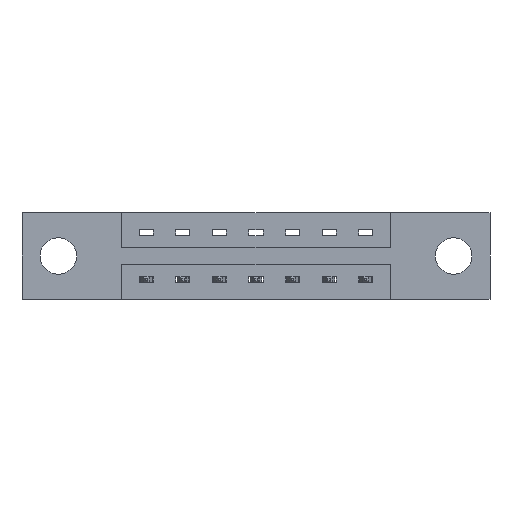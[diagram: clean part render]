
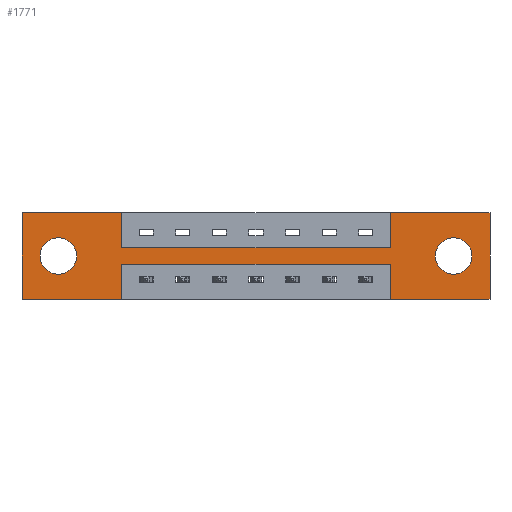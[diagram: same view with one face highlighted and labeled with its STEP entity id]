
A CAD part, front view. The second image highlights one B-rep face of the part: STEP entity #1771.
In plain terms, the highlighted planar face has unit normal (0, -1, 0).
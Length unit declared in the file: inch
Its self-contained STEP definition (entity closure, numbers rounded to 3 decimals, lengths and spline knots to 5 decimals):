
#3 = VERTEX_POINT ( 'NONE', #6277 ) ;
#59 = ORIENTED_EDGE ( 'NONE', *, *, #99, .F. ) ;
#99 = EDGE_CURVE ( 'NONE', #6538, #8846, #1955, .T. ) ;
#178 = AXIS2_PLACEMENT_3D ( 'NONE', #4753, #2896, #6939 ) ;
#201 = EDGE_CURVE ( 'NONE', #2395, #3969, #7067, .T. ) ;
#270 = ORIENTED_EDGE ( 'NONE', *, *, #6756, .T. ) ;
#272 = VECTOR ( 'NONE', #6194, 39.37008 ) ;
#516 = DIRECTION ( 'NONE',  ( 1., 0., 0. ) ) ;
#814 = EDGE_CURVE ( 'NONE', #7481, #3927, #6396, .T. ) ;
#838 = FACE_BOUND ( 'NONE', #1174, .T. ) ;
#1009 = CARTESIAN_POINT ( 'NONE',  ( 0.425, 0., 0. ) ) ;
#1174 = EDGE_LOOP ( 'NONE', ( #270, #1227 ) ) ;
#1227 = ORIENTED_EDGE ( 'NONE', *, *, #9350, .T. ) ;
#1290 = DIRECTION ( 'NONE',  ( 0., 0., -1. ) ) ;
#1318 = CARTESIAN_POINT ( 'NONE',  ( 0., 0., 0. ) ) ;
#1406 = VERTEX_POINT ( 'NONE', #3930 ) ;
#1412 = EDGE_CURVE ( 'NONE', #8813, #9386, #3619, .T. ) ;
#1627 = LINE ( 'NONE', #5317, #9279 ) ;
#1650 = CIRCLE ( 'NONE', #178, 0.078 ) ;
#1763 = CARTESIAN_POINT ( 'NONE',  ( 1.843, 0., -0.107 ) ) ;
#1771 = ADVANCED_FACE ( 'NONE', ( #838, #4845, #8669 ), #6172, .T. ) ;
#1793 = LINE ( 'NONE', #5709, #2046 ) ;
#1825 = CARTESIAN_POINT ( 'NONE',  ( 1.573, 0., -0.22 ) ) ;
#1839 = VERTEX_POINT ( 'NONE', #8819 ) ;
#1882 = VERTEX_POINT ( 'NONE', #7602 ) ;
#1948 = AXIS2_PLACEMENT_3D ( 'NONE', #8360, #5948, #5846 ) ;
#1955 = LINE ( 'NONE', #7317, #9540 ) ;
#1995 = VERTEX_POINT ( 'NONE', #5194 ) ;
#2046 = VECTOR ( 'NONE', #4275, 39.37008 ) ;
#2153 = VECTOR ( 'NONE', #2282, 39.37008 ) ;
#2155 = EDGE_CURVE ( 'NONE', #1882, #9260, #1650, .T. ) ;
#2158 = CARTESIAN_POINT ( 'NONE',  ( 0., 0., -0.37 ) ) ;
#2205 = ORIENTED_EDGE ( 'NONE', *, *, #6472, .F. ) ;
#2218 = CARTESIAN_POINT ( 'NONE',  ( 0., 0., 0. ) ) ;
#2282 = DIRECTION ( 'NONE',  ( -1., 0., 0. ) ) ;
#2288 = CARTESIAN_POINT ( 'NONE',  ( 0.155, 0., -0.185 ) ) ;
#2307 = CARTESIAN_POINT ( 'NONE',  ( 1.573, 0., -0.37 ) ) ;
#2395 = VERTEX_POINT ( 'NONE', #6501 ) ;
#2566 = ORIENTED_EDGE ( 'NONE', *, *, #2155, .T. ) ;
#2567 = DIRECTION ( 'NONE',  ( 0., 1., 0. ) ) ;
#2609 = CARTESIAN_POINT ( 'NONE',  ( 0.425, 0., -0.15 ) ) ;
#2838 = CIRCLE ( 'NONE', #5647, 0.078 ) ;
#2896 = DIRECTION ( 'NONE',  ( 0., 1., 0. ) ) ;
#2919 = EDGE_CURVE ( 'NONE', #1995, #6242, #9632, .T. ) ;
#3055 = DIRECTION ( 'NONE',  ( 0., 0., 1. ) ) ;
#3143 = VECTOR ( 'NONE', #8199, 39.37008 ) ;
#3165 = ORIENTED_EDGE ( 'NONE', *, *, #3813, .F. ) ;
#3193 = DIRECTION ( 'NONE',  ( 1., 0., 0. ) ) ;
#3371 = VECTOR ( 'NONE', #9126, 39.37008 ) ;
#3372 = EDGE_CURVE ( 'NONE', #8846, #1839, #9209, .T. ) ;
#3468 = CARTESIAN_POINT ( 'NONE',  ( 0.425, 0., -0.22 ) ) ;
#3476 = ORIENTED_EDGE ( 'NONE', *, *, #1412, .F. ) ;
#3619 = LINE ( 'NONE', #3981, #9204 ) ;
#3813 = EDGE_CURVE ( 'NONE', #1406, #2395, #1793, .T. ) ;
#3874 = VECTOR ( 'NONE', #7718, 39.37008 ) ;
#3924 = CIRCLE ( 'NONE', #1948, 0.078 ) ;
#3927 = VERTEX_POINT ( 'NONE', #9641 ) ;
#3930 = CARTESIAN_POINT ( 'NONE',  ( 1.573, 0., -0.15 ) ) ;
#3969 = VERTEX_POINT ( 'NONE', #8452 ) ;
#3981 = CARTESIAN_POINT ( 'NONE',  ( 0.425, 0., 0. ) ) ;
#4002 = CARTESIAN_POINT ( 'NONE',  ( 0.155, 0., -0.263 ) ) ;
#4010 = EDGE_LOOP ( 'NONE', ( #2566, #9467 ) ) ;
#4027 = CARTESIAN_POINT ( 'NONE',  ( 0., 0., 0. ) ) ;
#4216 = LINE ( 'NONE', #2158, #2153 ) ;
#4275 = DIRECTION ( 'NONE',  ( 0., 0., 1. ) ) ;
#4365 = EDGE_CURVE ( 'NONE', #1839, #7481, #4216, .T. ) ;
#4553 = LINE ( 'NONE', #2307, #272 ) ;
#4746 = CIRCLE ( 'NONE', #5968, 0.078 ) ;
#4753 = CARTESIAN_POINT ( 'NONE',  ( 0.155, 0., -0.185 ) ) ;
#4845 = FACE_BOUND ( 'NONE', #4010, .T. ) ;
#4879 = VECTOR ( 'NONE', #3193, 39.37008 ) ;
#5011 = LINE ( 'NONE', #2218, #3143 ) ;
#5044 = DIRECTION ( 'NONE',  ( 0., -1., 0. ) ) ;
#5111 = ORIENTED_EDGE ( 'NONE', *, *, #814, .F. ) ;
#5194 = CARTESIAN_POINT ( 'NONE',  ( 1.998, 0., -0.37 ) ) ;
#5252 = ORIENTED_EDGE ( 'NONE', *, *, #9171, .F. ) ;
#5317 = CARTESIAN_POINT ( 'NONE',  ( 0.425, 0., -0.15 ) ) ;
#5500 = ORIENTED_EDGE ( 'NONE', *, *, #3372, .F. ) ;
#5647 = AXIS2_PLACEMENT_3D ( 'NONE', #7125, #2567, #7844 ) ;
#5709 = CARTESIAN_POINT ( 'NONE',  ( 1.573, 0., 0. ) ) ;
#5846 = DIRECTION ( 'NONE',  ( 0., 0., -1. ) ) ;
#5948 = DIRECTION ( 'NONE',  ( 0., 1., 0. ) ) ;
#5968 = AXIS2_PLACEMENT_3D ( 'NONE', #2288, #7583, #3055 ) ;
#6167 = VECTOR ( 'NONE', #7612, 39.37008 ) ;
#6172 = PLANE ( 'NONE',  #8748 ) ;
#6194 = DIRECTION ( 'NONE',  ( 0., 0., 1. ) ) ;
#6235 = DIRECTION ( 'NONE',  ( 0., 0., -1. ) ) ;
#6242 = VERTEX_POINT ( 'NONE', #9678 ) ;
#6277 = CARTESIAN_POINT ( 'NONE',  ( 1.843, 0., -0.263 ) ) ;
#6315 = CARTESIAN_POINT ( 'NONE',  ( 0., 0., -0.37 ) ) ;
#6396 = LINE ( 'NONE', #4027, #6167 ) ;
#6472 = EDGE_CURVE ( 'NONE', #3969, #1995, #8400, .T. ) ;
#6501 = CARTESIAN_POINT ( 'NONE',  ( 1.573, 0., 0. ) ) ;
#6512 = DIRECTION ( 'NONE',  ( 0., 0., -1. ) ) ;
#6538 = VERTEX_POINT ( 'NONE', #1825 ) ;
#6558 = VERTEX_POINT ( 'NONE', #1763 ) ;
#6560 = VECTOR ( 'NONE', #6235, 39.37008 ) ;
#6584 = EDGE_LOOP ( 'NONE', ( #5500, #59, #5252, #9177, #2205, #7580, #3165, #7571, #3476, #6649, #5111, #8598 ) ) ;
#6649 = ORIENTED_EDGE ( 'NONE', *, *, #8458, .F. ) ;
#6756 = EDGE_CURVE ( 'NONE', #6558, #3, #3924, .T. ) ;
#6939 = DIRECTION ( 'NONE',  ( 0., 0., 1. ) ) ;
#7067 = LINE ( 'NONE', #1318, #4879 ) ;
#7125 = CARTESIAN_POINT ( 'NONE',  ( 1.843, 0., -0.185 ) ) ;
#7205 = CARTESIAN_POINT ( 'NONE',  ( 0.425, 0., -0.37 ) ) ;
#7278 = CARTESIAN_POINT ( 'NONE',  ( 0., 0., -0.37 ) ) ;
#7317 = CARTESIAN_POINT ( 'NONE',  ( 0.425, 0., -0.22 ) ) ;
#7481 = VERTEX_POINT ( 'NONE', #9534 ) ;
#7571 = ORIENTED_EDGE ( 'NONE', *, *, #9071, .F. ) ;
#7580 = ORIENTED_EDGE ( 'NONE', *, *, #201, .F. ) ;
#7583 = DIRECTION ( 'NONE',  ( 0., 1., 0. ) ) ;
#7602 = CARTESIAN_POINT ( 'NONE',  ( 0.155, 0., -0.107 ) ) ;
#7612 = DIRECTION ( 'NONE',  ( 0., 0., 1. ) ) ;
#7718 = DIRECTION ( 'NONE',  ( -1., 0., 0. ) ) ;
#7844 = DIRECTION ( 'NONE',  ( 0., 0., -1. ) ) ;
#8199 = DIRECTION ( 'NONE',  ( 1., 0., 0. ) ) ;
#8356 = CARTESIAN_POINT ( 'NONE',  ( 1.998, 0., 0. ) ) ;
#8360 = CARTESIAN_POINT ( 'NONE',  ( 1.843, 0., -0.185 ) ) ;
#8400 = LINE ( 'NONE', #8356, #6560 ) ;
#8452 = CARTESIAN_POINT ( 'NONE',  ( 1.998, 0., 0. ) ) ;
#8458 = EDGE_CURVE ( 'NONE', #3927, #8813, #5011, .T. ) ;
#8480 = EDGE_CURVE ( 'NONE', #9260, #1882, #4746, .T. ) ;
#8598 = ORIENTED_EDGE ( 'NONE', *, *, #4365, .F. ) ;
#8669 = FACE_OUTER_BOUND ( 'NONE', #6584, .T. ) ;
#8748 = AXIS2_PLACEMENT_3D ( 'NONE', #6315, #5044, #6512 ) ;
#8813 = VERTEX_POINT ( 'NONE', #1009 ) ;
#8819 = CARTESIAN_POINT ( 'NONE',  ( 0.425, 0., -0.37 ) ) ;
#8846 = VERTEX_POINT ( 'NONE', #3468 ) ;
#9071 = EDGE_CURVE ( 'NONE', #9386, #1406, #1627, .T. ) ;
#9126 = DIRECTION ( 'NONE',  ( 0., 0., -1. ) ) ;
#9171 = EDGE_CURVE ( 'NONE', #6242, #6538, #4553, .T. ) ;
#9177 = ORIENTED_EDGE ( 'NONE', *, *, #2919, .F. ) ;
#9204 = VECTOR ( 'NONE', #1290, 39.37008 ) ;
#9209 = LINE ( 'NONE', #7205, #3371 ) ;
#9260 = VERTEX_POINT ( 'NONE', #4002 ) ;
#9279 = VECTOR ( 'NONE', #516, 39.37008 ) ;
#9350 = EDGE_CURVE ( 'NONE', #3, #6558, #2838, .T. ) ;
#9386 = VERTEX_POINT ( 'NONE', #2609 ) ;
#9467 = ORIENTED_EDGE ( 'NONE', *, *, #8480, .T. ) ;
#9534 = CARTESIAN_POINT ( 'NONE',  ( 0., 0., -0.37 ) ) ;
#9540 = VECTOR ( 'NONE', #9586, 39.37008 ) ;
#9586 = DIRECTION ( 'NONE',  ( -1., 0., 0. ) ) ;
#9632 = LINE ( 'NONE', #7278, #3874 ) ;
#9641 = CARTESIAN_POINT ( 'NONE',  ( 0., 0., 0. ) ) ;
#9678 = CARTESIAN_POINT ( 'NONE',  ( 1.573, 0., -0.37 ) ) ;
